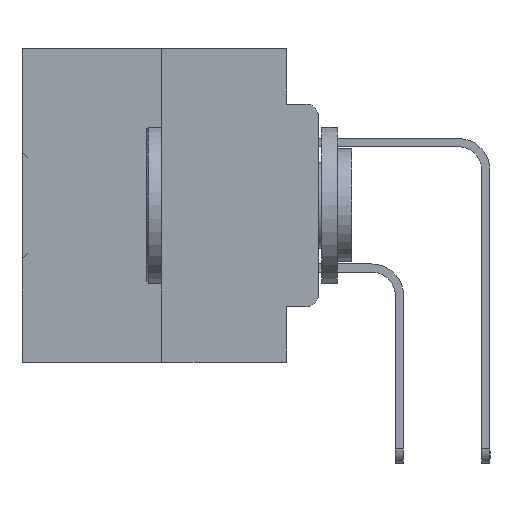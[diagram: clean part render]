
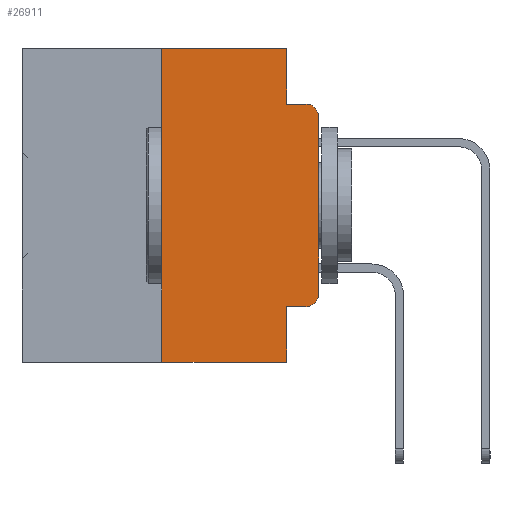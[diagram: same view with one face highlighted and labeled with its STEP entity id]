
A CAD part, left-side view. The second image highlights one B-rep face of the part: STEP entity #26911.
In plain terms, the highlighted planar face has unit normal (-1, 0, 0).
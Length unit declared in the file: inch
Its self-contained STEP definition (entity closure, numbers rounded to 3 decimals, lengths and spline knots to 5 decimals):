
#610 = PLANE ( 'NONE',  #21649 ) ;
#633 = LINE ( 'NONE', #20665, #3212 ) ;
#1036 = CARTESIAN_POINT ( 'NONE',  ( 0., 0.051, 0. ) ) ;
#1077 = VERTEX_POINT ( 'NONE', #2518 ) ;
#1295 = AXIS2_PLACEMENT_3D ( 'NONE', #30037, #27142, #35260 ) ;
#1302 = EDGE_CURVE ( 'NONE', #12548, #33762, #28343, .T. ) ;
#1685 = ORIENTED_EDGE ( 'NONE', *, *, #33545, .F. ) ;
#1924 = VERTEX_POINT ( 'NONE', #20472 ) ;
#2443 = CARTESIAN_POINT ( 'NONE',  ( 0., 0.051, -0.5 ) ) ;
#2459 = DIRECTION ( 'NONE',  ( 0., -1., 0. ) ) ;
#2518 = CARTESIAN_POINT ( 'NONE',  ( 0., 0.25, -0.5 ) ) ;
#3212 = VECTOR ( 'NONE', #17956, 39.37008 ) ;
#3469 = ORIENTED_EDGE ( 'NONE', *, *, #13445, .F. ) ;
#3968 = CARTESIAN_POINT ( 'NONE',  ( 0., 0.473, -0.5 ) ) ;
#4711 = EDGE_CURVE ( 'NONE', #1924, #25948, #633, .T. ) ;
#4734 = DIRECTION ( 'NONE',  ( 0., -1., 0. ) ) ;
#6017 = CARTESIAN_POINT ( 'NONE',  ( 0., 0.051, -0.4115 ) ) ;
#6131 = CARTESIAN_POINT ( 'NONE',  ( 0., 0.473, 0. ) ) ;
#8067 = VERTEX_POINT ( 'NONE', #10500 ) ;
#8330 = CARTESIAN_POINT ( 'NONE',  ( 0., 0.25, 0. ) ) ;
#8465 = CIRCLE ( 'NONE', #20273, 0.02 ) ;
#8601 = ORIENTED_EDGE ( 'NONE', *, *, #24520, .T. ) ;
#9075 = VECTOR ( 'NONE', #33135, 39.37008 ) ;
#9528 = DIRECTION ( 'NONE',  ( 0., 0., -1. ) ) ;
#10148 = ORIENTED_EDGE ( 'NONE', *, *, #28015, .T. ) ;
#10418 = EDGE_CURVE ( 'NONE', #8067, #1924, #29676, .T. ) ;
#10500 = CARTESIAN_POINT ( 'NONE',  ( 0., 0.25, 0. ) ) ;
#10656 = CARTESIAN_POINT ( 'NONE',  ( 0., 0.051, -0.4115 ) ) ;
#10907 = ORIENTED_EDGE ( 'NONE', *, *, #4711, .F. ) ;
#11135 = VERTEX_POINT ( 'NONE', #33880 ) ;
#11986 = VECTOR ( 'NONE', #37233, 39.37008 ) ;
#12503 = VERTEX_POINT ( 'NONE', #35411 ) ;
#12548 = VERTEX_POINT ( 'NONE', #20496 ) ;
#13317 = VERTEX_POINT ( 'NONE', #10656 ) ;
#13445 = EDGE_CURVE ( 'NONE', #1077, #8067, #26438, .T. ) ;
#14692 = VECTOR ( 'NONE', #4734, 39.37008 ) ;
#14717 = LINE ( 'NONE', #29116, #25159 ) ;
#15200 = CARTESIAN_POINT ( 'NONE',  ( 0., 0.473, 0. ) ) ;
#15211 = VECTOR ( 'NONE', #18736, 39.37008 ) ;
#17956 = DIRECTION ( 'NONE',  ( 0., 0., -1. ) ) ;
#18022 = EDGE_LOOP ( 'NONE', ( #35758, #8601, #28257, #10907, #23819, #3469, #21354, #1685, #18167, #10148 ) ) ;
#18167 = ORIENTED_EDGE ( 'NONE', *, *, #28885, .T. ) ;
#18736 = DIRECTION ( 'NONE',  ( 0., 0., -1. ) ) ;
#19089 = VERTEX_POINT ( 'NONE', #2443 ) ;
#19594 = CARTESIAN_POINT ( 'NONE',  ( 0., 0., 0. ) ) ;
#20273 = AXIS2_PLACEMENT_3D ( 'NONE', #26775, #35854, #24424 ) ;
#20472 = CARTESIAN_POINT ( 'NONE',  ( 0., 0.051, 0. ) ) ;
#20496 = CARTESIAN_POINT ( 'NONE',  ( 0., 0., -0.3915 ) ) ;
#20665 = CARTESIAN_POINT ( 'NONE',  ( 0., 0.051, 0. ) ) ;
#21354 = ORIENTED_EDGE ( 'NONE', *, *, #24705, .T. ) ;
#21649 = AXIS2_PLACEMENT_3D ( 'NONE', #15200, #35954, #9528 ) ;
#21671 = VECTOR ( 'NONE', #23331, 39.37008 ) ;
#23106 = EDGE_CURVE ( 'NONE', #25948, #11135, #14717, .T. ) ;
#23331 = DIRECTION ( 'NONE',  ( 0., 0., 1. ) ) ;
#23363 = LINE ( 'NONE', #6017, #33598 ) ;
#23819 = ORIENTED_EDGE ( 'NONE', *, *, #10418, .F. ) ;
#24424 = DIRECTION ( 'NONE',  ( 0., 0., -1. ) ) ;
#24520 = EDGE_CURVE ( 'NONE', #33762, #11135, #8465, .T. ) ;
#24705 = EDGE_CURVE ( 'NONE', #1077, #19089, #37177, .T. ) ;
#25159 = VECTOR ( 'NONE', #2459, 39.37008 ) ;
#25948 = VERTEX_POINT ( 'NONE', #26632 ) ;
#26438 = LINE ( 'NONE', #8330, #21671 ) ;
#26632 = CARTESIAN_POINT ( 'NONE',  ( 0., 0.051, -0.0885 ) ) ;
#26775 = CARTESIAN_POINT ( 'NONE',  ( 0., 0.02, -0.1085 ) ) ;
#26798 = CIRCLE ( 'NONE', #1295, 0.02 ) ;
#26911 = ADVANCED_FACE ( 'NONE', ( #32481 ), #610, .F. ) ;
#27142 = DIRECTION ( 'NONE',  ( -1., 0., 0. ) ) ;
#28015 = EDGE_CURVE ( 'NONE', #12503, #12548, #26798, .T. ) ;
#28257 = ORIENTED_EDGE ( 'NONE', *, *, #23106, .F. ) ;
#28343 = LINE ( 'NONE', #19594, #11986 ) ;
#28885 = EDGE_CURVE ( 'NONE', #13317, #12503, #23363, .T. ) ;
#29116 = CARTESIAN_POINT ( 'NONE',  ( 0., 0.051, -0.0885 ) ) ;
#29676 = LINE ( 'NONE', #6131, #9075 ) ;
#29964 = CARTESIAN_POINT ( 'NONE',  ( 0., 0., -0.1085 ) ) ;
#30037 = CARTESIAN_POINT ( 'NONE',  ( 0., 0.02, -0.3915 ) ) ;
#32481 = FACE_OUTER_BOUND ( 'NONE', #18022, .T. ) ;
#33135 = DIRECTION ( 'NONE',  ( 0., -1., 0. ) ) ;
#33545 = EDGE_CURVE ( 'NONE', #13317, #19089, #36751, .T. ) ;
#33598 = VECTOR ( 'NONE', #35163, 39.37008 ) ;
#33762 = VERTEX_POINT ( 'NONE', #29964 ) ;
#33880 = CARTESIAN_POINT ( 'NONE',  ( 0., 0.02, -0.0885 ) ) ;
#35163 = DIRECTION ( 'NONE',  ( 0., -1., 0. ) ) ;
#35260 = DIRECTION ( 'NONE',  ( 0., 0., -1. ) ) ;
#35411 = CARTESIAN_POINT ( 'NONE',  ( 0., 0.02, -0.4115 ) ) ;
#35758 = ORIENTED_EDGE ( 'NONE', *, *, #1302, .T. ) ;
#35854 = DIRECTION ( 'NONE',  ( -1., 0., 0. ) ) ;
#35954 = DIRECTION ( 'NONE',  ( 1., 0., 0. ) ) ;
#36751 = LINE ( 'NONE', #1036, #15211 ) ;
#37177 = LINE ( 'NONE', #3968, #14692 ) ;
#37233 = DIRECTION ( 'NONE',  ( 0., 0., 1. ) ) ;
